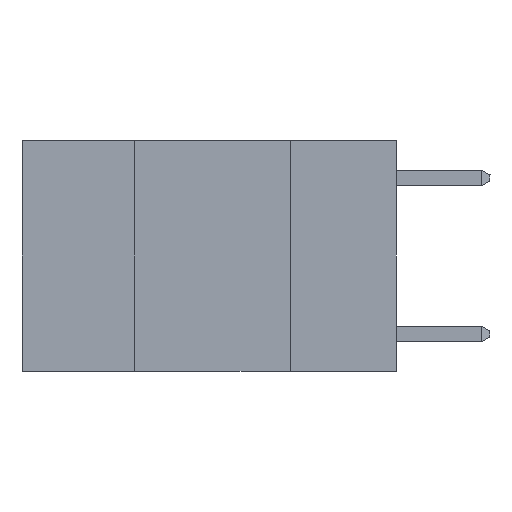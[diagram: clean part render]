
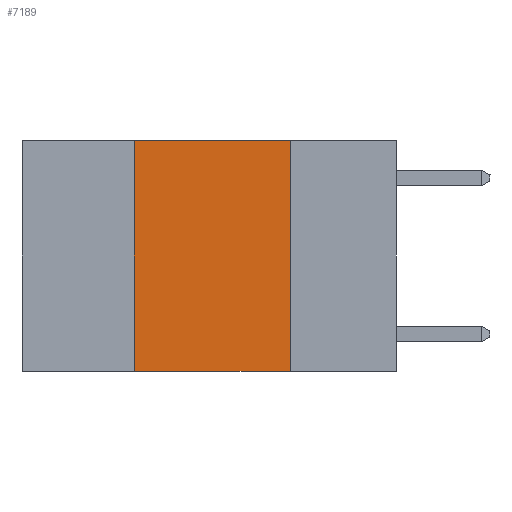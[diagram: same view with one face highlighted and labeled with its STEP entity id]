
A CAD part, left-side view. The second image highlights one B-rep face of the part: STEP entity #7189.
In plain terms, the highlighted planar face has unit normal (-1, 0, 0).
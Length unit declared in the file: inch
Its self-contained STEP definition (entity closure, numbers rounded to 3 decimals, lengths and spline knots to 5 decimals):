
#325 = LINE ( 'NONE', #2579, #13737 ) ;
#357 = LINE ( 'NONE', #7615, #8146 ) ;
#476 = CARTESIAN_POINT ( 'NONE',  ( 0., 0.17, 0. ) ) ;
#655 = ORIENTED_EDGE ( 'NONE', *, *, #4342, .F. ) ;
#1444 = CARTESIAN_POINT ( 'NONE',  ( 0., 0.17, -0.37 ) ) ;
#1769 = DIRECTION ( 'NONE',  ( 0., 0., -1. ) ) ;
#1856 = VERTEX_POINT ( 'NONE', #9262 ) ;
#2394 = AXIS2_PLACEMENT_3D ( 'NONE', #15026, #7357, #16299 ) ;
#2407 = EDGE_LOOP ( 'NONE', ( #7058, #8575, #655, #7390 ) ) ;
#2579 = CARTESIAN_POINT ( 'NONE',  ( 0., 0.42, 0. ) ) ;
#2986 = VECTOR ( 'NONE', #1769, 39.37008 ) ;
#3225 = VERTEX_POINT ( 'NONE', #1444 ) ;
#3919 = EDGE_CURVE ( 'NONE', #1856, #3225, #13371, .T. ) ;
#4342 = EDGE_CURVE ( 'NONE', #12206, #5096, #325, .T. ) ;
#4856 = CARTESIAN_POINT ( 'NONE',  ( 0., 0.42, -0.37 ) ) ;
#5096 = VERTEX_POINT ( 'NONE', #8283 ) ;
#5734 = LINE ( 'NONE', #8296, #8831 ) ;
#6962 = DIRECTION ( 'NONE',  ( 0., -1., 0. ) ) ;
#7058 = ORIENTED_EDGE ( 'NONE', *, *, #3919, .F. ) ;
#7189 = ADVANCED_FACE ( 'NONE', ( #10099 ), #9950, .F. ) ;
#7357 = DIRECTION ( 'NONE',  ( 1., 0., 0. ) ) ;
#7390 = ORIENTED_EDGE ( 'NONE', *, *, #9951, .T. ) ;
#7615 = CARTESIAN_POINT ( 'NONE',  ( 0., 0.6, -0.37 ) ) ;
#8146 = VECTOR ( 'NONE', #15276, 39.37008 ) ;
#8283 = CARTESIAN_POINT ( 'NONE',  ( 0., 0.42, 0. ) ) ;
#8296 = CARTESIAN_POINT ( 'NONE',  ( 0., 0.6, 0. ) ) ;
#8575 = ORIENTED_EDGE ( 'NONE', *, *, #15221, .F. ) ;
#8831 = VECTOR ( 'NONE', #6962, 39.37008 ) ;
#9262 = CARTESIAN_POINT ( 'NONE',  ( 0., 0.17, 0. ) ) ;
#9950 = PLANE ( 'NONE',  #2394 ) ;
#9951 = EDGE_CURVE ( 'NONE', #12206, #3225, #357, .T. ) ;
#10099 = FACE_OUTER_BOUND ( 'NONE', #2407, .T. ) ;
#10451 = DIRECTION ( 'NONE',  ( 0., 0., 1. ) ) ;
#12206 = VERTEX_POINT ( 'NONE', #4856 ) ;
#13371 = LINE ( 'NONE', #476, #2986 ) ;
#13737 = VECTOR ( 'NONE', #10451, 39.37008 ) ;
#15026 = CARTESIAN_POINT ( 'NONE',  ( 0., 0.6, 0. ) ) ;
#15221 = EDGE_CURVE ( 'NONE', #5096, #1856, #5734, .T. ) ;
#15276 = DIRECTION ( 'NONE',  ( 0., -1., 0. ) ) ;
#16299 = DIRECTION ( 'NONE',  ( 0., 0., -1. ) ) ;
